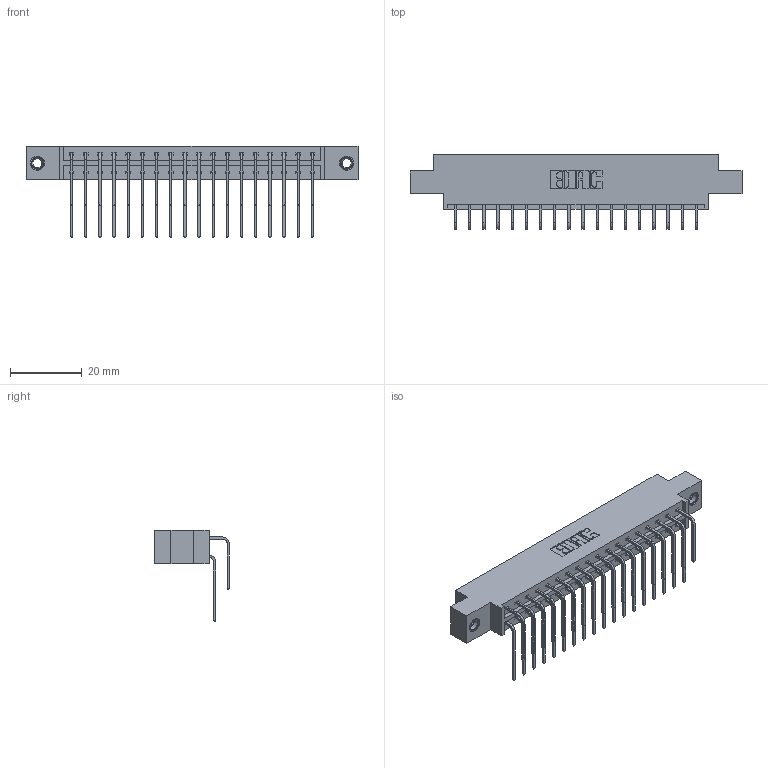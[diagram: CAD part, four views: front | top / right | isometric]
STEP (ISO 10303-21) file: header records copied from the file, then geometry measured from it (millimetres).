
FILE_DESCRIPTION (( 'STEP AP203' ), '1' );
FILE_NAME ('833-036-559-807.STEP', '2020-06-03T04:21:11', ( '' ), ( '' ), 'SwSTEP 2.0', 'SolidWorks 2020', '' );
FILE_SCHEMA (( 'CONFIG_CONTROL_DESIGN' ));
Length unit declared in the file: inch
Products named in the file (5): 345-292-001_558 559 Tail - 1; 833 Part_Offset - .156 Dia - TI; 345-250-001_345-250-005-103; 833-036-559-807; 345-292-001_559 Tail - 2
Assembly tree (39 placements, depth 2):
  833-036-559-807
    833 Part_Offset - .156 Dia - TI
    345-292-001_558 559 Tail - 1  x18
    345-292-001_559 Tail - 2  x18
    345-250-001_345-250-005-103  x2
Bounding box: 92.86 x 20.9 x 25.53 mm (x, y, z)
Volume: 9222.6 mm3; surface area: 11935 mm2
Topology: 39 solids, 39 shells, 2122 faces, 6255 edges, 4114 vertices
Faces by surface type: plane 1474, cylinder 632, cone 12, torus 4
Entity records: 17786 total; most frequent: CARTESIAN_POINT 3012, ORIENTED_EDGE 2890, DIRECTION 2627, EDGE_CURVE 1445, LINE 1257, VECTOR 1257, VERTEX_POINT 956, AXIS2_PLACEMENT_3D 685
